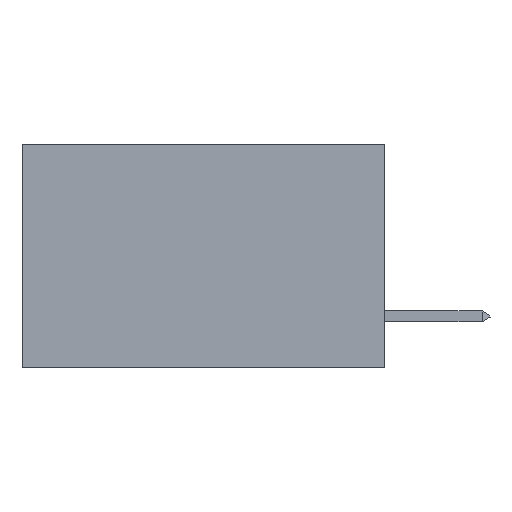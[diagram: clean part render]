
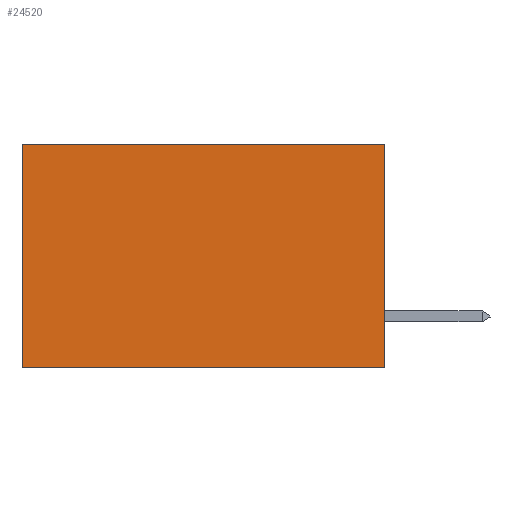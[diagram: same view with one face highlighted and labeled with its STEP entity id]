
A CAD part, left-side view. The second image highlights one B-rep face of the part: STEP entity #24520.
In plain terms, the highlighted planar face has unit normal (-1, 0, 0).
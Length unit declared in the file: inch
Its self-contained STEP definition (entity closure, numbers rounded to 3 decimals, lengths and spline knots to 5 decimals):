
#2398 = VECTOR ( 'NONE', #22806, 39.37008 ) ;
#3068 = VECTOR ( 'NONE', #21266, 39.37008 ) ;
#3420 = VERTEX_POINT ( 'NONE', #7645 ) ;
#3515 = ORIENTED_EDGE ( 'NONE', *, *, #13306, .T. ) ;
#4018 = VECTOR ( 'NONE', #16713, 39.37008 ) ;
#4647 = LINE ( 'NONE', #6712, #4018 ) ;
#5872 = DIRECTION ( 'NONE',  ( 0., 0., -1. ) ) ;
#6014 = ORIENTED_EDGE ( 'NONE', *, *, #25745, .T. ) ;
#6712 = CARTESIAN_POINT ( 'NONE',  ( 0.2875, 0., -0.37 ) ) ;
#7645 = CARTESIAN_POINT ( 'NONE',  ( 0.2875, 0.6, -0.37 ) ) ;
#8438 = CARTESIAN_POINT ( 'NONE',  ( 0.2875, 0., 0. ) ) ;
#8475 = CARTESIAN_POINT ( 'NONE',  ( 0.2875, 0.6, 0. ) ) ;
#8949 = DIRECTION ( 'NONE',  ( 0., 0., -1. ) ) ;
#8952 = ORIENTED_EDGE ( 'NONE', *, *, #9809, .F. ) ;
#9447 = VERTEX_POINT ( 'NONE', #8475 ) ;
#9809 = EDGE_CURVE ( 'NONE', #18847, #3420, #4647, .T. ) ;
#11003 = VECTOR ( 'NONE', #5872, 39.37008 ) ;
#13050 = PLANE ( 'NONE',  #14418 ) ;
#13306 = EDGE_CURVE ( 'NONE', #9447, #3420, #24453, .T. ) ;
#13554 = EDGE_CURVE ( 'NONE', #22468, #18847, #13567, .T. ) ;
#13567 = LINE ( 'NONE', #8438, #2398 ) ;
#14418 = AXIS2_PLACEMENT_3D ( 'NONE', #25212, #25383, #8949 ) ;
#16713 = DIRECTION ( 'NONE',  ( 0., 1., 0. ) ) ;
#17049 = CARTESIAN_POINT ( 'NONE',  ( 0.2875, 0., 0. ) ) ;
#17734 = LINE ( 'NONE', #17049, #3068 ) ;
#17738 = ORIENTED_EDGE ( 'NONE', *, *, #13554, .F. ) ;
#18847 = VERTEX_POINT ( 'NONE', #22939 ) ;
#19900 = CARTESIAN_POINT ( 'NONE',  ( 0.2875, 0., 0. ) ) ;
#20656 = FACE_OUTER_BOUND ( 'NONE', #26514, .T. ) ;
#21266 = DIRECTION ( 'NONE',  ( 0., 1., 0. ) ) ;
#22468 = VERTEX_POINT ( 'NONE', #19900 ) ;
#22806 = DIRECTION ( 'NONE',  ( 0., 0., -1. ) ) ;
#22939 = CARTESIAN_POINT ( 'NONE',  ( 0.2875, 0., -0.37 ) ) ;
#24108 = CARTESIAN_POINT ( 'NONE',  ( 0.2875, 0.6, 0. ) ) ;
#24453 = LINE ( 'NONE', #24108, #11003 ) ;
#24520 = ADVANCED_FACE ( 'NONE', ( #20656 ), #13050, .F. ) ;
#25212 = CARTESIAN_POINT ( 'NONE',  ( 0.2875, 0., 0. ) ) ;
#25383 = DIRECTION ( 'NONE',  ( 1., 0., 0. ) ) ;
#25745 = EDGE_CURVE ( 'NONE', #22468, #9447, #17734, .T. ) ;
#26514 = EDGE_LOOP ( 'NONE', ( #3515, #8952, #17738, #6014 ) ) ;
